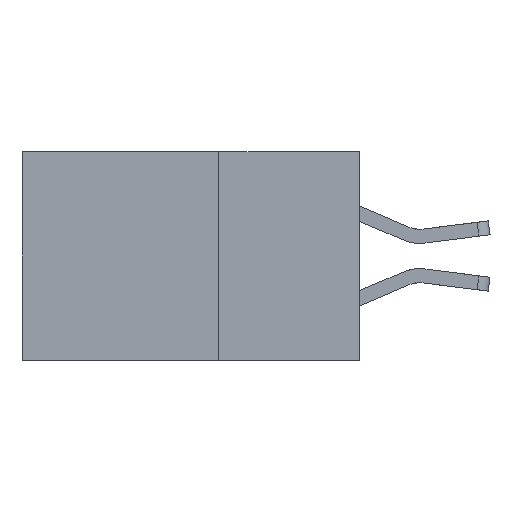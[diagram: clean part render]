
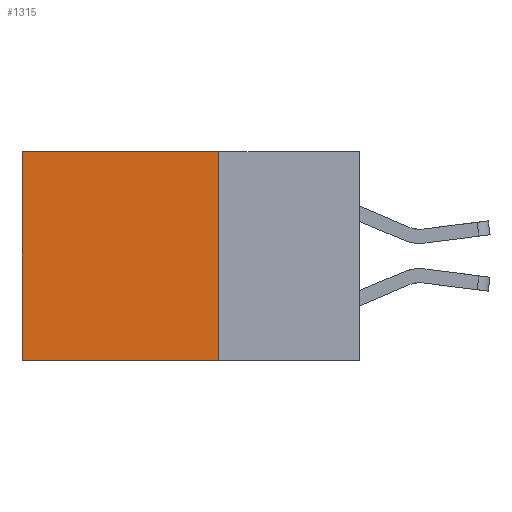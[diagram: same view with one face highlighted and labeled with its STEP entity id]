
A CAD part, left-side view. The second image highlights one B-rep face of the part: STEP entity #1315.
In plain terms, the highlighted planar face has unit normal (-1, 0, 0).
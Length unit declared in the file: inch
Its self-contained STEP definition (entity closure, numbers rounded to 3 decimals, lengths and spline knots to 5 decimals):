
#770 = CARTESIAN_POINT ( 'NONE',  ( 0.2875, 0.25, 0. ) ) ;
#814 = CARTESIAN_POINT ( 'NONE',  ( 0.2875, 0.6, 0. ) ) ;
#1296 = ORIENTED_EDGE ( 'NONE', *, *, #3636, .T. ) ;
#1315 = ADVANCED_FACE ( 'NONE', ( #2867 ), #4754, .F. ) ;
#1497 = ORIENTED_EDGE ( 'NONE', *, *, #5243, .F. ) ;
#2867 = FACE_OUTER_BOUND ( 'NONE', #8196, .T. ) ;
#3632 = VECTOR ( 'NONE', #11401, 39.37008 ) ;
#3636 = EDGE_CURVE ( 'NONE', #11021, #7248, #9439, .T. ) ;
#3780 = EDGE_CURVE ( 'NONE', #10101, #11021, #11704, .T. ) ;
#3783 = CARTESIAN_POINT ( 'NONE',  ( 0.2875, 0.25, 0. ) ) ;
#4672 = VECTOR ( 'NONE', #8348, 39.37008 ) ;
#4754 = PLANE ( 'NONE',  #11429 ) ;
#5136 = ORIENTED_EDGE ( 'NONE', *, *, #7867, .F. ) ;
#5243 = EDGE_CURVE ( 'NONE', #10101, #5952, #5342, .T. ) ;
#5342 = LINE ( 'NONE', #10385, #4672 ) ;
#5413 = LINE ( 'NONE', #7629, #7942 ) ;
#5867 = DIRECTION ( 'NONE',  ( 0., 1., 0. ) ) ;
#5952 = VERTEX_POINT ( 'NONE', #9286 ) ;
#6481 = CARTESIAN_POINT ( 'NONE',  ( 0.2875, 0.6, 0. ) ) ;
#6740 = CARTESIAN_POINT ( 'NONE',  ( 0.2875, 0.25, 0. ) ) ;
#7248 = VERTEX_POINT ( 'NONE', #12361 ) ;
#7629 = CARTESIAN_POINT ( 'NONE',  ( 0.2875, 0.25, -0.37 ) ) ;
#7750 = ORIENTED_EDGE ( 'NONE', *, *, #3780, .T. ) ;
#7867 = EDGE_CURVE ( 'NONE', #5952, #7248, #5413, .T. ) ;
#7942 = VECTOR ( 'NONE', #11631, 39.37008 ) ;
#8196 = EDGE_LOOP ( 'NONE', ( #1296, #5136, #1497, #7750 ) ) ;
#8348 = DIRECTION ( 'NONE',  ( 0., 0., -1. ) ) ;
#8864 = DIRECTION ( 'NONE',  ( 1., 0., 0. ) ) ;
#9286 = CARTESIAN_POINT ( 'NONE',  ( 0.2875, 0.25, -0.37 ) ) ;
#9439 = LINE ( 'NONE', #6481, #3632 ) ;
#10101 = VERTEX_POINT ( 'NONE', #6740 ) ;
#10385 = CARTESIAN_POINT ( 'NONE',  ( 0.2875, 0.25, 0. ) ) ;
#11021 = VERTEX_POINT ( 'NONE', #814 ) ;
#11401 = DIRECTION ( 'NONE',  ( 0., 0., -1. ) ) ;
#11429 = AXIS2_PLACEMENT_3D ( 'NONE', #3783, #8864, #11872 ) ;
#11631 = DIRECTION ( 'NONE',  ( 0., 1., 0. ) ) ;
#11704 = LINE ( 'NONE', #770, #12396 ) ;
#11872 = DIRECTION ( 'NONE',  ( 0., 0., -1. ) ) ;
#12361 = CARTESIAN_POINT ( 'NONE',  ( 0.2875, 0.6, -0.37 ) ) ;
#12396 = VECTOR ( 'NONE', #5867, 39.37008 ) ;
